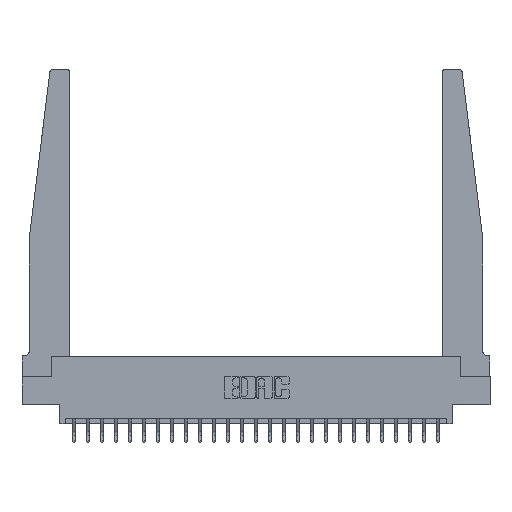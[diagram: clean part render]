
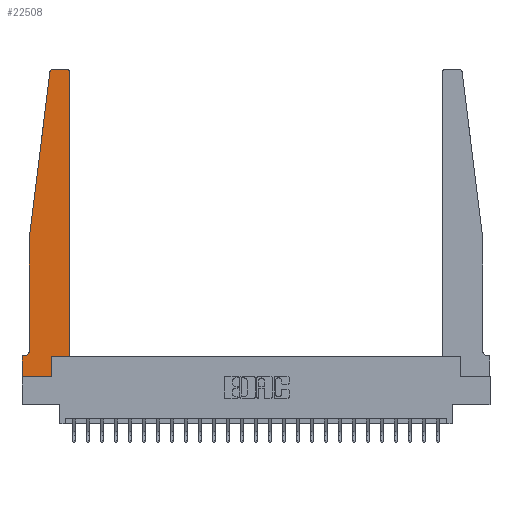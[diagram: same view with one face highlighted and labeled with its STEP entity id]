
A CAD part, top view. The second image highlights one B-rep face of the part: STEP entity #22508.
In plain terms, the highlighted planar face has unit normal (0, 0, 1).
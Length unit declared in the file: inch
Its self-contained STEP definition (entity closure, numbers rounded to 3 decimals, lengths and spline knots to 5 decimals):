
#341 = CARTESIAN_POINT ( 'NONE',  ( 0.425, 0.18, 0.37 ) ) ;
#408 = CARTESIAN_POINT ( 'NONE',  ( 0.425, 0.18, 0.37 ) ) ;
#707 = ORIENTED_EDGE ( 'NONE', *, *, #17584, .T. ) ;
#1048 = DIRECTION ( 'NONE',  ( -0.122, -0.992, 0. ) ) ;
#1144 = VERTEX_POINT ( 'NONE', #10833 ) ;
#1757 = VERTEX_POINT ( 'NONE', #16561 ) ;
#2337 = DIRECTION ( 'NONE',  ( 1., 0., 0. ) ) ;
#2677 = VERTEX_POINT ( 'NONE', #11657 ) ;
#2689 = LINE ( 'NONE', #3625, #17401 ) ;
#2978 = CARTESIAN_POINT ( 'NONE',  ( 0.065, 0.1875, 0.37 ) ) ;
#3003 = CARTESIAN_POINT ( 'NONE',  ( 0.2605, 0.18, 0.37 ) ) ;
#3041 = DIRECTION ( 'NONE',  ( 1., 0., 0. ) ) ;
#3058 = DIRECTION ( 'NONE',  ( -1., 0., 0. ) ) ;
#3132 = EDGE_CURVE ( 'NONE', #19597, #8973, #23254, .T. ) ;
#3135 = ORIENTED_EDGE ( 'NONE', *, *, #19378, .T. ) ;
#3625 = CARTESIAN_POINT ( 'NONE',  ( 0.25, 2.75, 0.37 ) ) ;
#3862 = VECTOR ( 'NONE', #23694, 39.37008 ) ;
#4215 = CARTESIAN_POINT ( 'NONE',  ( 0.27653, 2.72, 0.37 ) ) ;
#4627 = ORIENTED_EDGE ( 'NONE', *, *, #14780, .T. ) ;
#4672 = AXIS2_PLACEMENT_3D ( 'NONE', #17060, #5567, #18980 ) ;
#5315 = DIRECTION ( 'NONE',  ( 1., 0., 0. ) ) ;
#5375 = CARTESIAN_POINT ( 'NONE',  ( 0.395, 2.75, 0.37 ) ) ;
#5567 = DIRECTION ( 'NONE',  ( 0., 0., -1. ) ) ;
#5575 = DIRECTION ( 'NONE',  ( -1., 0., 0. ) ) ;
#5652 = LINE ( 'NONE', #408, #14121 ) ;
#5776 = FACE_OUTER_BOUND ( 'NONE', #22555, .T. ) ;
#6040 = AXIS2_PLACEMENT_3D ( 'NONE', #18313, #14614, #3041 ) ;
#6181 = DIRECTION ( 'NONE',  ( 1., 0., 0. ) ) ;
#6267 = CARTESIAN_POINT ( 'NONE',  ( 0.065, 1.25, 0.37 ) ) ;
#6364 = VECTOR ( 'NONE', #18944, 39.37008 ) ;
#6463 = ORIENTED_EDGE ( 'NONE', *, *, #15844, .T. ) ;
#6484 = LINE ( 'NONE', #23976, #11011 ) ;
#6848 = EDGE_CURVE ( 'NONE', #8189, #1144, #18084, .T. ) ;
#7947 = CARTESIAN_POINT ( 'NONE',  ( 0.24675, 2.72367, 0.37 ) ) ;
#8189 = VERTEX_POINT ( 'NONE', #24368 ) ;
#8299 = EDGE_CURVE ( 'NONE', #8973, #11723, #2689, .T. ) ;
#8578 = ORIENTED_EDGE ( 'NONE', *, *, #8299, .T. ) ;
#8973 = VERTEX_POINT ( 'NONE', #5375 ) ;
#9060 = CARTESIAN_POINT ( 'NONE',  ( 0., 0., 0.37 ) ) ;
#9412 = CARTESIAN_POINT ( 'NONE',  ( 0.395, 2.72, 0.37 ) ) ;
#9536 = VERTEX_POINT ( 'NONE', #20939 ) ;
#10734 = PLANE ( 'NONE',  #6040 ) ;
#10833 = CARTESIAN_POINT ( 'NONE',  ( 0.2605, 0., 0.37 ) ) ;
#11011 = VECTOR ( 'NONE', #1048, 39.37008 ) ;
#11382 = DIRECTION ( 'NONE',  ( 1., 0., 0. ) ) ;
#11657 = CARTESIAN_POINT ( 'NONE',  ( 0., 0.1875, 0.37 ) ) ;
#11718 = EDGE_CURVE ( 'NONE', #22862, #24334, #6484, .T. ) ;
#11723 = VERTEX_POINT ( 'NONE', #16348 ) ;
#12206 = VECTOR ( 'NONE', #16443, 39.37008 ) ;
#12243 = ORIENTED_EDGE ( 'NONE', *, *, #6848, .T. ) ;
#12448 = CARTESIAN_POINT ( 'NONE',  ( 0.425, 2.72, 0.37 ) ) ;
#12457 = VECTOR ( 'NONE', #5315, 39.37008 ) ;
#12661 = EDGE_CURVE ( 'NONE', #1144, #9536, #12786, .T. ) ;
#12786 = LINE ( 'NONE', #3003, #12206 ) ;
#13298 = VECTOR ( 'NONE', #3058, 39.37008 ) ;
#13432 = ORIENTED_EDGE ( 'NONE', *, *, #3132, .T. ) ;
#13609 = EDGE_CURVE ( 'NONE', #11723, #22862, #13965, .T. ) ;
#13703 = ORIENTED_EDGE ( 'NONE', *, *, #13609, .T. ) ;
#13867 = DIRECTION ( 'NONE',  ( 0., 1., 0. ) ) ;
#13965 = CIRCLE ( 'NONE', #18127, 0.03 ) ;
#14121 = VECTOR ( 'NONE', #2337, 39.37008 ) ;
#14164 = LINE ( 'NONE', #21807, #3862 ) ;
#14614 = DIRECTION ( 'NONE',  ( 0., 0., 1. ) ) ;
#14780 = EDGE_CURVE ( 'NONE', #24334, #20504, #21037, .T. ) ;
#15184 = EDGE_CURVE ( 'NONE', #16478, #2677, #22175, .T. ) ;
#15844 = EDGE_CURVE ( 'NONE', #2677, #8189, #14164, .T. ) ;
#16064 = ORIENTED_EDGE ( 'NONE', *, *, #15184, .T. ) ;
#16348 = CARTESIAN_POINT ( 'NONE',  ( 0.27653, 2.75, 0.37 ) ) ;
#16443 = DIRECTION ( 'NONE',  ( 0., 1., 0. ) ) ;
#16478 = VERTEX_POINT ( 'NONE', #21529 ) ;
#16561 = CARTESIAN_POINT ( 'NONE',  ( 0.425, 0.18, 0.37 ) ) ;
#17026 = CARTESIAN_POINT ( 'NONE',  ( 0.065, 1.25, 0.37 ) ) ;
#17060 = CARTESIAN_POINT ( 'NONE',  ( 0.015, 0.2375, 0.37 ) ) ;
#17079 = CIRCLE ( 'NONE', #4672, 0.05 ) ;
#17256 = ORIENTED_EDGE ( 'NONE', *, *, #12661, .T. ) ;
#17401 = VECTOR ( 'NONE', #5575, 39.37008 ) ;
#17584 = EDGE_CURVE ( 'NONE', #20504, #16478, #17079, .T. ) ;
#17648 = DIRECTION ( 'NONE',  ( 0., 0., 1. ) ) ;
#17851 = ORIENTED_EDGE ( 'NONE', *, *, #24507, .T. ) ;
#18084 = LINE ( 'NONE', #9060, #12457 ) ;
#18127 = AXIS2_PLACEMENT_3D ( 'NONE', #4215, #17648, #6181 ) ;
#18313 = CARTESIAN_POINT ( 'NONE',  ( 0., 0.1875, 0.37 ) ) ;
#18944 = DIRECTION ( 'NONE',  ( 0., -1., 0. ) ) ;
#18980 = DIRECTION ( 'NONE',  ( -1., 0., 0. ) ) ;
#19331 = ORIENTED_EDGE ( 'NONE', *, *, #11718, .T. ) ;
#19378 = EDGE_CURVE ( 'NONE', #1757, #19597, #24407, .T. ) ;
#19380 = VECTOR ( 'NONE', #13867, 39.37008 ) ;
#19597 = VERTEX_POINT ( 'NONE', #12448 ) ;
#20504 = VERTEX_POINT ( 'NONE', #24570 ) ;
#20939 = CARTESIAN_POINT ( 'NONE',  ( 0.2605, 0.18, 0.37 ) ) ;
#21037 = LINE ( 'NONE', #17026, #6364 ) ;
#21529 = CARTESIAN_POINT ( 'NONE',  ( 0.015, 0.1875, 0.37 ) ) ;
#21807 = CARTESIAN_POINT ( 'NONE',  ( 0., 0., 0.37 ) ) ;
#21958 = AXIS2_PLACEMENT_3D ( 'NONE', #9412, #22740, #11382 ) ;
#22175 = LINE ( 'NONE', #2978, #13298 ) ;
#22508 = ADVANCED_FACE ( 'NONE', ( #5776 ), #10734, .T. ) ;
#22555 = EDGE_LOOP ( 'NONE', ( #8578, #13703, #19331, #4627, #707, #16064, #6463, #12243, #17256, #17851, #3135, #13432 ) ) ;
#22740 = DIRECTION ( 'NONE',  ( 0., 0., 1. ) ) ;
#22862 = VERTEX_POINT ( 'NONE', #7947 ) ;
#23254 = CIRCLE ( 'NONE', #21958, 0.03 ) ;
#23694 = DIRECTION ( 'NONE',  ( 0., -1., 0. ) ) ;
#23976 = CARTESIAN_POINT ( 'NONE',  ( 0.065, 1.25, 0.37 ) ) ;
#24334 = VERTEX_POINT ( 'NONE', #6267 ) ;
#24368 = CARTESIAN_POINT ( 'NONE',  ( 0., 0., 0.37 ) ) ;
#24407 = LINE ( 'NONE', #341, #19380 ) ;
#24507 = EDGE_CURVE ( 'NONE', #9536, #1757, #5652, .T. ) ;
#24570 = CARTESIAN_POINT ( 'NONE',  ( 0.065, 0.2375, 0.37 ) ) ;
